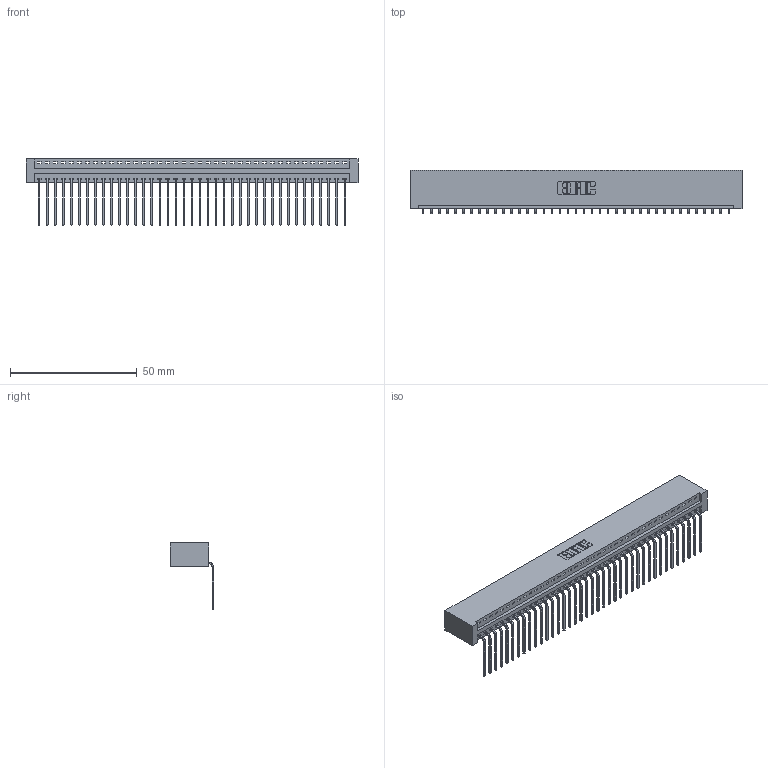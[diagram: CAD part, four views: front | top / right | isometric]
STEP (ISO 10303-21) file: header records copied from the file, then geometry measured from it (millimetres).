
FILE_DESCRIPTION (( 'STEP AP203' ), '1' );
FILE_NAME ('346-039-559-101.STEP', '2022-05-07T08:04:15', ( '' ), ( '' ), 'SwSTEP 2.0', 'SolidWorks 2020', '' );
FILE_SCHEMA (( 'CONFIG_CONTROL_DESIGN' ));
Length unit declared in the file: inch
Products named in the file (3): 346 Part_No Mounting Lugs; 346-039-559-101; 345-292-001_558 559 Tail - 1
Assembly tree (40 placements, depth 2):
  346-039-559-101
    346 Part_No Mounting Lugs
    345-292-001_558 559 Tail - 1  x39
Bounding box: 131.06 x 17.08 x 26.16 mm (x, y, z)
Volume: 13204.4 mm3; surface area: 17321.7 mm2
Topology: 40 solids, 40 shells, 2454 faces, 7403 edges, 4882 vertices
Faces by surface type: plane 1710, cylinder 744
Entity records: 24415 total; most frequent: CARTESIAN_POINT 4193, ORIENTED_EDGE 4166, DIRECTION 3697, EDGE_CURVE 2083, VECTOR 1803, LINE 1803, VERTEX_POINT 1386, AXIS2_PLACEMENT_3D 947
